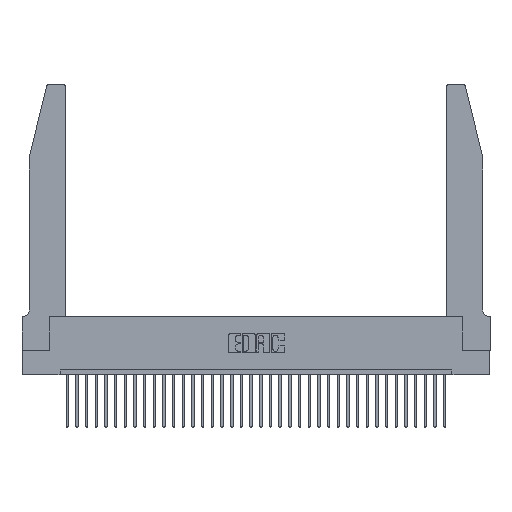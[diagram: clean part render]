
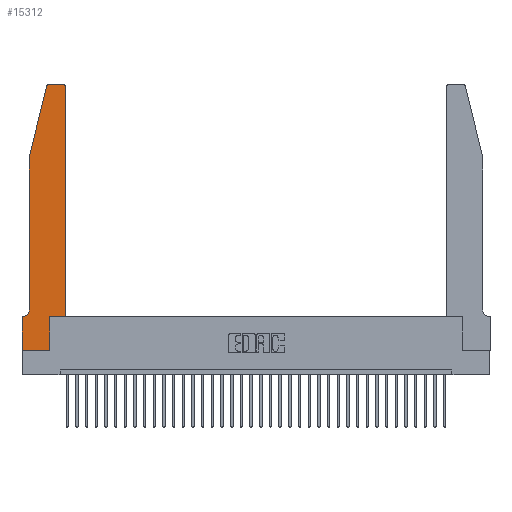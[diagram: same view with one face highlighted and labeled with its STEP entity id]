
A CAD part, top view. The second image highlights one B-rep face of the part: STEP entity #15312.
In plain terms, the highlighted planar face has unit normal (0, 0, 1).
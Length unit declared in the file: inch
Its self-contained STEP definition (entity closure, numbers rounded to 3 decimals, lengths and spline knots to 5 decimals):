
#648 = LINE ( 'NONE', #938, #25745 ) ;
#938 = CARTESIAN_POINT ( 'NONE',  ( 0.4505, 0.35, 0.37 ) ) ;
#1008 = EDGE_CURVE ( 'NONE', #34541, #15734, #19423, .T. ) ;
#1665 = DIRECTION ( 'NONE',  ( 0., 0., 1. ) ) ;
#1829 = LINE ( 'NONE', #19540, #14068 ) ;
#3154 = CIRCLE ( 'NONE', #7066, 0.03 ) ;
#3478 = EDGE_CURVE ( 'NONE', #14112, #11192, #11194, .T. ) ;
#3878 = EDGE_CURVE ( 'NONE', #17188, #4943, #31467, .T. ) ;
#4024 = CARTESIAN_POINT ( 'NONE',  ( 0.4205, 2.75, 0.37 ) ) ;
#4668 = CARTESIAN_POINT ( 'NONE',  ( 0.0755, 0.42, 0.37 ) ) ;
#4943 = VERTEX_POINT ( 'NONE', #4024 ) ;
#5128 = CARTESIAN_POINT ( 'NONE',  ( 0.4505, 0.35, 0.37 ) ) ;
#5672 = VECTOR ( 'NONE', #33048, 39.37008 ) ;
#5741 = DIRECTION ( 'NONE',  ( -1., 0., 0. ) ) ;
#5761 = ORIENTED_EDGE ( 'NONE', *, *, #10950, .T. ) ;
#5789 = EDGE_LOOP ( 'NONE', ( #5761, #6156, #31414, #32960, #16594, #27997, #31462, #30770, #29232, #8307, #33798, #11542 ) ) ;
#6156 = ORIENTED_EDGE ( 'NONE', *, *, #7226, .T. ) ;
#6521 = CARTESIAN_POINT ( 'NONE',  ( 0.2605, 2.75, 0.37 ) ) ;
#6806 = VECTOR ( 'NONE', #26709, 39.37008 ) ;
#7066 = AXIS2_PLACEMENT_3D ( 'NONE', #12283, #25410, #25540 ) ;
#7226 = EDGE_CURVE ( 'NONE', #24571, #16834, #3154, .T. ) ;
#7254 = CARTESIAN_POINT ( 'NONE',  ( 0.4205, 2.72, 0.37 ) ) ;
#8307 = ORIENTED_EDGE ( 'NONE', *, *, #1008, .T. ) ;
#8589 = CARTESIAN_POINT ( 'NONE',  ( 0.4505, 2.72, 0.37 ) ) ;
#8674 = CARTESIAN_POINT ( 'NONE',  ( 0.0755, 0.35, 0.37 ) ) ;
#9315 = VECTOR ( 'NONE', #27551, 39.37008 ) ;
#9643 = EDGE_CURVE ( 'NONE', #16834, #14112, #31484, .T. ) ;
#9864 = CARTESIAN_POINT ( 'NONE',  ( 0.2865, 0., 0.37 ) ) ;
#10950 = EDGE_CURVE ( 'NONE', #4943, #24571, #30776, .T. ) ;
#11085 = CARTESIAN_POINT ( 'NONE',  ( 0., 0., 0.37 ) ) ;
#11192 = VERTEX_POINT ( 'NONE', #4668 ) ;
#11194 = LINE ( 'NONE', #13834, #5672 ) ;
#11506 = VECTOR ( 'NONE', #23796, 39.37008 ) ;
#11542 = ORIENTED_EDGE ( 'NONE', *, *, #3878, .T. ) ;
#12283 = CARTESIAN_POINT ( 'NONE',  ( 0.284, 2.72, 0.37 ) ) ;
#13207 = DIRECTION ( 'NONE',  ( 1., 0., 0. ) ) ;
#13566 = DIRECTION ( 'NONE',  ( 1., 0., 0. ) ) ;
#13601 = EDGE_CURVE ( 'NONE', #32079, #14365, #1829, .T. ) ;
#13834 = CARTESIAN_POINT ( 'NONE',  ( 0.0755, 2., 0.37 ) ) ;
#13845 = EDGE_CURVE ( 'NONE', #32844, #32079, #22549, .T. ) ;
#14068 = VECTOR ( 'NONE', #14233, 39.37008 ) ;
#14112 = VERTEX_POINT ( 'NONE', #30236 ) ;
#14233 = DIRECTION ( 'NONE',  ( 0., -1., 0. ) ) ;
#14365 = VERTEX_POINT ( 'NONE', #11085 ) ;
#14686 = CARTESIAN_POINT ( 'NONE',  ( 0.284, 2.75, 0.37 ) ) ;
#15312 = ADVANCED_FACE ( 'NONE', ( #27143 ), #17960, .T. ) ;
#15734 = VERTEX_POINT ( 'NONE', #28492 ) ;
#16144 = CARTESIAN_POINT ( 'NONE',  ( 0., 0., 0.37 ) ) ;
#16594 = ORIENTED_EDGE ( 'NONE', *, *, #24021, .T. ) ;
#16687 = AXIS2_PLACEMENT_3D ( 'NONE', #21047, #29281, #13566 ) ;
#16760 = CARTESIAN_POINT ( 'NONE',  ( 0.2865, 0.35, 0.37 ) ) ;
#16834 = VERTEX_POINT ( 'NONE', #34119 ) ;
#16906 = EDGE_CURVE ( 'NONE', #15734, #17188, #648, .T. ) ;
#17188 = VERTEX_POINT ( 'NONE', #8589 ) ;
#17394 = CARTESIAN_POINT ( 'NONE',  ( 0., 0.35, 0.37 ) ) ;
#17808 = CIRCLE ( 'NONE', #20987, 0.07 ) ;
#17956 = CARTESIAN_POINT ( 'NONE',  ( 0.0755, 2., 0.37 ) ) ;
#17960 = PLANE ( 'NONE',  #16687 ) ;
#19423 = LINE ( 'NONE', #5128, #22435 ) ;
#19540 = CARTESIAN_POINT ( 'NONE',  ( 0., 0., 0.37 ) ) ;
#19657 = DIRECTION ( 'NONE',  ( 0., 1., 0. ) ) ;
#20589 = AXIS2_PLACEMENT_3D ( 'NONE', #7254, #1665, #22160 ) ;
#20987 = AXIS2_PLACEMENT_3D ( 'NONE', #29963, #24635, #5741 ) ;
#21047 = CARTESIAN_POINT ( 'NONE',  ( 0., 0.35, 0.37 ) ) ;
#21407 = CARTESIAN_POINT ( 'NONE',  ( 0.0055, 0.35, 0.37 ) ) ;
#21508 = DIRECTION ( 'NONE',  ( -1., 0., 0. ) ) ;
#21827 = EDGE_CURVE ( 'NONE', #30306, #34541, #23333, .T. ) ;
#22160 = DIRECTION ( 'NONE',  ( 1., 0., 0. ) ) ;
#22435 = VECTOR ( 'NONE', #13207, 39.37008 ) ;
#22549 = LINE ( 'NONE', #8674, #33592 ) ;
#23333 = LINE ( 'NONE', #16760, #9315 ) ;
#23796 = DIRECTION ( 'NONE',  ( -0.239, -0.971, 0. ) ) ;
#24021 = EDGE_CURVE ( 'NONE', #11192, #32844, #17808, .T. ) ;
#24043 = VECTOR ( 'NONE', #25750, 39.37008 ) ;
#24571 = VERTEX_POINT ( 'NONE', #14686 ) ;
#24635 = DIRECTION ( 'NONE',  ( 0., 0., -1. ) ) ;
#25410 = DIRECTION ( 'NONE',  ( 0., 0., 1. ) ) ;
#25540 = DIRECTION ( 'NONE',  ( 1., 0., 0. ) ) ;
#25745 = VECTOR ( 'NONE', #19657, 39.37008 ) ;
#25750 = DIRECTION ( 'NONE',  ( -1., 0., 0. ) ) ;
#26709 = DIRECTION ( 'NONE',  ( 1., 0., 0. ) ) ;
#27143 = FACE_OUTER_BOUND ( 'NONE', #5789, .T. ) ;
#27551 = DIRECTION ( 'NONE',  ( 0., 1., 0. ) ) ;
#27997 = ORIENTED_EDGE ( 'NONE', *, *, #13845, .T. ) ;
#28492 = CARTESIAN_POINT ( 'NONE',  ( 0.4505, 0.35, 0.37 ) ) ;
#28638 = CARTESIAN_POINT ( 'NONE',  ( 0.2865, 0.35, 0.37 ) ) ;
#29232 = ORIENTED_EDGE ( 'NONE', *, *, #21827, .T. ) ;
#29281 = DIRECTION ( 'NONE',  ( 0., 0., 1. ) ) ;
#29963 = CARTESIAN_POINT ( 'NONE',  ( 0.0055, 0.42, 0.37 ) ) ;
#30236 = CARTESIAN_POINT ( 'NONE',  ( 0.0755, 2., 0.37 ) ) ;
#30306 = VERTEX_POINT ( 'NONE', #9864 ) ;
#30770 = ORIENTED_EDGE ( 'NONE', *, *, #33088, .T. ) ;
#30776 = LINE ( 'NONE', #6521, #24043 ) ;
#30978 = LINE ( 'NONE', #16144, #6806 ) ;
#31414 = ORIENTED_EDGE ( 'NONE', *, *, #9643, .T. ) ;
#31462 = ORIENTED_EDGE ( 'NONE', *, *, #13601, .T. ) ;
#31467 = CIRCLE ( 'NONE', #20589, 0.03 ) ;
#31484 = LINE ( 'NONE', #17956, #11506 ) ;
#32079 = VERTEX_POINT ( 'NONE', #17394 ) ;
#32844 = VERTEX_POINT ( 'NONE', #21407 ) ;
#32960 = ORIENTED_EDGE ( 'NONE', *, *, #3478, .T. ) ;
#33048 = DIRECTION ( 'NONE',  ( 0., -1., 0. ) ) ;
#33088 = EDGE_CURVE ( 'NONE', #14365, #30306, #30978, .T. ) ;
#33592 = VECTOR ( 'NONE', #21508, 39.37008 ) ;
#33798 = ORIENTED_EDGE ( 'NONE', *, *, #16906, .T. ) ;
#34119 = CARTESIAN_POINT ( 'NONE',  ( 0.25487, 2.72718, 0.37 ) ) ;
#34541 = VERTEX_POINT ( 'NONE', #28638 ) ;
